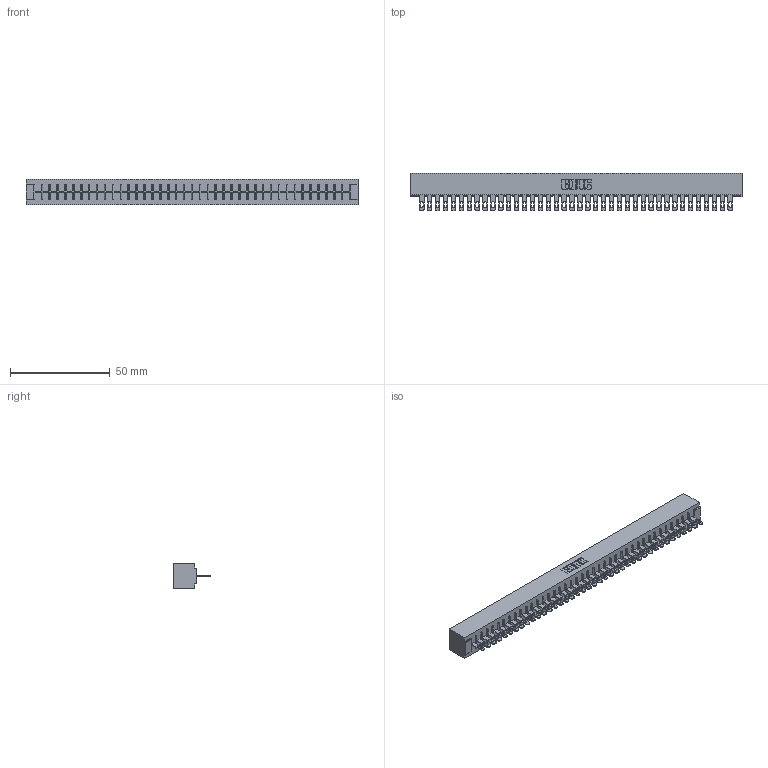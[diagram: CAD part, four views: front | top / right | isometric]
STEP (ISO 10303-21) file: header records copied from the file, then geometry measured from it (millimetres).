
FILE_DESCRIPTION (( 'STEP AP203' ), '1' );
FILE_NAME ('316-040-500-101.STEP', '2018-07-31T05:14:52', ( '' ), ( '' ), 'SwSTEP 2.0', 'SolidWorks 2016', '' );
FILE_SCHEMA (( 'CONFIG_CONTROL_DESIGN' ));
Length unit declared in the file: inch
Products named in the file (3): 306 Part_No Mounting; 306-290-001_100; 316-040-500-101
Assembly tree (41 placements, depth 2):
  316-040-500-101
    306 Part_No Mounting
    306-290-001_100  x40
Bounding box: 166.37 x 18.87 x 12.7 mm (x, y, z)
Volume: 19096.4 mm3; surface area: 20412.2 mm2
Topology: 41 solids, 41 shells, 3148 faces, 8892 edges, 5712 vertices
Faces by surface type: plane 2064, cylinder 924, sphere 160
Entity records: 37447 total; most frequent: CARTESIAN_POINT 6287, ORIENTED_EDGE 6232, DIRECTION 6200, EDGE_CURVE 3116, LINE 2438, VECTOR 2438, VERTEX_POINT 1968, AXIS2_PLACEMENT_3D 1881
